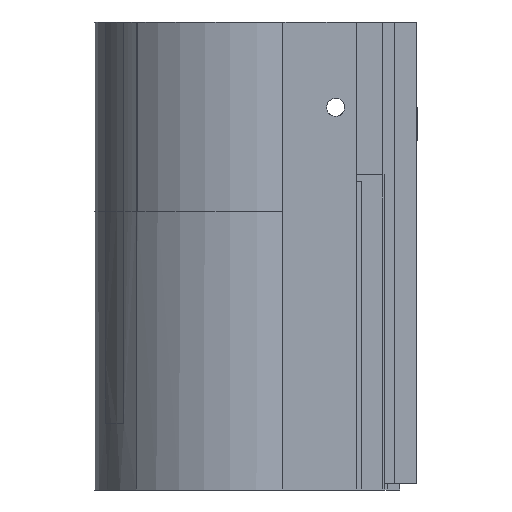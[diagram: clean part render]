
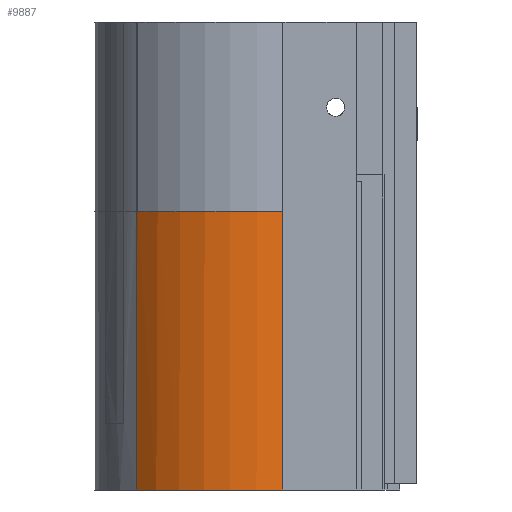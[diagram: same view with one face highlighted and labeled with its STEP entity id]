
A CAD part, left-side view. The second image highlights one B-rep face of the part: STEP entity #9887.
In plain terms, the highlighted cylindrical face has radius 25.3 mm (diameter 50.6 mm), a partial arc.
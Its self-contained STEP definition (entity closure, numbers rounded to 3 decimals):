
#1326 = CYLINDRICAL_SURFACE('',#1327,25.3);
#1327 = AXIS2_PLACEMENT_3D('',#1328,#1329,#1330);
#1328 = CARTESIAN_POINT('',(0.,17.3,45.));
#1329 = DIRECTION('',(0.,0.,1.));
#1330 = DIRECTION('',(1.,0.,0.));
#1355 = PLANE('',#1356);
#1356 = AXIS2_PLACEMENT_3D('',#1357,#1358,#1359);
#1357 = CARTESIAN_POINT('',(-11.232,-5.37,-1.));
#1358 = DIRECTION('',(0.,0.,1.));
#1359 = DIRECTION('',(1.,0.,0.));
#4476 = VERTEX_POINT('',#4477);
#4477 = CARTESIAN_POINT('',(-17.45,35.619,45.));
#4504 = EDGE_CURVE('',#4476,#4505,#4507,.T.);
#4505 = VERTEX_POINT('',#4506);
#4506 = CARTESIAN_POINT('',(-17.45,35.619,-1.));
#4507 = SURFACE_CURVE('',#4508,(#4512,#4519),.PCURVE_S1.);
#4508 = LINE('',#4509,#4510);
#4509 = CARTESIAN_POINT('',(-17.45,35.619,76.2));
#4510 = VECTOR('',#4511,1.);
#4511 = DIRECTION('',(0.,0.,-1.));
#4512 = PCURVE('',#1326,#4513);
#4513 = DEFINITIONAL_REPRESENTATION('',(#4514),#4518);
#4514 = LINE('',#4515,#4516);
#4515 = CARTESIAN_POINT('',(-3.951,31.2));
#4516 = VECTOR('',#4517,1.);
#4517 = DIRECTION('',(0.,-1.));
#4518 = ( GEOMETRIC_REPRESENTATION_CONTEXT(2) 
PARAMETRIC_REPRESENTATION_CONTEXT() REPRESENTATION_CONTEXT('2D SPACE',''
  ) );
#4519 = PCURVE('',#4520,#4525);
#4520 = CYLINDRICAL_SURFACE('',#4521,25.3);
#4521 = AXIS2_PLACEMENT_3D('',#4522,#4523,#4524);
#4522 = CARTESIAN_POINT('',(0.,17.3,45.));
#4523 = DIRECTION('',(0.,0.,1.));
#4524 = DIRECTION('',(1.,0.,0.));
#4525 = DEFINITIONAL_REPRESENTATION('',(#4526),#4530);
#4526 = LINE('',#4527,#4528);
#4527 = CARTESIAN_POINT('',(-3.951,31.2));
#4528 = VECTOR('',#4529,1.);
#4529 = DIRECTION('',(0.,-1.));
#4530 = ( GEOMETRIC_REPRESENTATION_CONTEXT(2) 
PARAMETRIC_REPRESENTATION_CONTEXT() REPRESENTATION_CONTEXT('2D SPACE',''
  ) );
#4862 = EDGE_CURVE('',#4863,#4505,#4865,.T.);
#4863 = VERTEX_POINT('',#4864);
#4864 = CARTESIAN_POINT('',(-24.618,11.467,-1.));
#4865 = SURFACE_CURVE('',#4866,(#4871,#4882),.PCURVE_S1.);
#4866 = CIRCLE('',#4867,25.3);
#4867 = AXIS2_PLACEMENT_3D('',#4868,#4869,#4870);
#4868 = CARTESIAN_POINT('',(0.,17.3,-1.));
#4869 = DIRECTION('',(0.,0.,-1.));
#4870 = DIRECTION('',(1.,0.,0.));
#4871 = PCURVE('',#1355,#4872);
#4872 = DEFINITIONAL_REPRESENTATION('',(#4873),#4881);
#4873 = ( BOUNDED_CURVE() B_SPLINE_CURVE(2,(#4874,#4875,#4876,#4877,
#4878,#4879,#4880),.UNSPECIFIED.,.T.,.F.) B_SPLINE_CURVE_WITH_KNOTS((1,2
    ,2,2,2,1),(-2.094,0.,2.094,4.189,
6.283,8.378),.UNSPECIFIED.) CURVE() 
GEOMETRIC_REPRESENTATION_ITEM() RATIONAL_B_SPLINE_CURVE((1.,0.5,1.,0.5,
1.,0.5,1.)) REPRESENTATION_ITEM('') );
#4874 = CARTESIAN_POINT('',(36.532,22.67));
#4875 = CARTESIAN_POINT('',(36.532,-21.151));
#4876 = CARTESIAN_POINT('',(-1.418,0.76));
#4877 = CARTESIAN_POINT('',(-39.368,22.67));
#4878 = CARTESIAN_POINT('',(-1.418,44.581));
#4879 = CARTESIAN_POINT('',(36.532,66.491));
#4880 = CARTESIAN_POINT('',(36.532,22.67));
#4881 = ( GEOMETRIC_REPRESENTATION_CONTEXT(2) 
PARAMETRIC_REPRESENTATION_CONTEXT() REPRESENTATION_CONTEXT('2D SPACE',''
  ) );
#4882 = PCURVE('',#4520,#4883);
#4883 = DEFINITIONAL_REPRESENTATION('',(#4884),#4888);
#4884 = LINE('',#4885,#4886);
#4885 = CARTESIAN_POINT('',(0.,-46.));
#4886 = VECTOR('',#4887,1.);
#4887 = DIRECTION('',(-1.,0.));
#4888 = ( GEOMETRIC_REPRESENTATION_CONTEXT(2) 
PARAMETRIC_REPRESENTATION_CONTEXT() REPRESENTATION_CONTEXT('2D SPACE',''
  ) );
#4906 = PLANE('',#4907);
#4907 = AXIS2_PLACEMENT_3D('',#4908,#4909,#4910);
#4908 = CARTESIAN_POINT('',(-11.993,11.467,-1.));
#4909 = DIRECTION('',(0.,-1.,0.));
#4910 = DIRECTION('',(-1.,0.,0.));
#9847 = CYLINDRICAL_SURFACE('',#9848,25.3);
#9848 = AXIS2_PLACEMENT_3D('',#9849,#9850,#9851);
#9849 = CARTESIAN_POINT('',(0.,17.3,45.));
#9850 = DIRECTION('',(0.,0.,-1.));
#9851 = DIRECTION('',(1.,0.,0.));
#9887 = ADVANCED_FACE('',(#9888),#4520,.T.);
#9888 = FACE_BOUND('',#9889,.F.);
#9889 = EDGE_LOOP('',(#9890,#9921,#9940,#9941,#9942));
#9890 = ORIENTED_EDGE('',*,*,#9891,.T.);
#9891 = EDGE_CURVE('',#9892,#9894,#9896,.T.);
#9892 = VERTEX_POINT('',#9893);
#9893 = CARTESIAN_POINT('',(-17.662,35.415,45.));
#9894 = VERTEX_POINT('',#9895);
#9895 = CARTESIAN_POINT('',(-24.618,11.467,45.));
#9896 = SURFACE_CURVE('',#9897,(#9902,#9909),.PCURVE_S1.);
#9897 = CIRCLE('',#9898,25.3);
#9898 = AXIS2_PLACEMENT_3D('',#9899,#9900,#9901);
#9899 = CARTESIAN_POINT('',(0.,17.3,45.));
#9900 = DIRECTION('',(0.,0.,1.));
#9901 = DIRECTION('',(1.,0.,0.));
#9902 = PCURVE('',#4520,#9903);
#9903 = DEFINITIONAL_REPRESENTATION('',(#9904),#9908);
#9904 = LINE('',#9905,#9906);
#9905 = CARTESIAN_POINT('',(-6.283,0.));
#9906 = VECTOR('',#9907,1.);
#9907 = DIRECTION('',(1.,0.));
#9908 = ( GEOMETRIC_REPRESENTATION_CONTEXT(2) 
PARAMETRIC_REPRESENTATION_CONTEXT() REPRESENTATION_CONTEXT('2D SPACE',''
  ) );
#9909 = PCURVE('',#9910,#9915);
#9910 = CYLINDRICAL_SURFACE('',#9911,25.3);
#9911 = AXIS2_PLACEMENT_3D('',#9912,#9913,#9914);
#9912 = CARTESIAN_POINT('',(0.,17.3,45.));
#9913 = DIRECTION('',(0.,0.,-1.));
#9914 = DIRECTION('',(1.,0.,0.));
#9915 = DEFINITIONAL_REPRESENTATION('',(#9916),#9920);
#9916 = LINE('',#9917,#9918);
#9917 = CARTESIAN_POINT('',(0.,0.));
#9918 = VECTOR('',#9919,1.);
#9919 = DIRECTION('',(-1.,0.));
#9920 = ( GEOMETRIC_REPRESENTATION_CONTEXT(2) 
PARAMETRIC_REPRESENTATION_CONTEXT() REPRESENTATION_CONTEXT('2D SPACE',''
  ) );
#9921 = ORIENTED_EDGE('',*,*,#9922,.F.);
#9922 = EDGE_CURVE('',#4863,#9894,#9923,.T.);
#9923 = SURFACE_CURVE('',#9924,(#9928,#9934),.PCURVE_S1.);
#9924 = LINE('',#9925,#9926);
#9925 = CARTESIAN_POINT('',(-24.618,11.467,45.));
#9926 = VECTOR('',#9927,1.);
#9927 = DIRECTION('',(0.,0.,1.));
#9928 = PCURVE('',#4520,#9929);
#9929 = DEFINITIONAL_REPRESENTATION('',(#9930),#9933);
#9930 = B_SPLINE_CURVE_WITH_KNOTS('',1,(#9931,#9932),.UNSPECIFIED.,.F.,
  .F.,(2,2),(-46.,0.),.PIECEWISE_BEZIER_KNOTS.);
#9931 = CARTESIAN_POINT('',(-2.909,-46.));
#9932 = CARTESIAN_POINT('',(-2.909,0.));
#9933 = ( GEOMETRIC_REPRESENTATION_CONTEXT(2) 
PARAMETRIC_REPRESENTATION_CONTEXT() REPRESENTATION_CONTEXT('2D SPACE',''
  ) );
#9934 = PCURVE('',#4906,#9935);
#9935 = DEFINITIONAL_REPRESENTATION('',(#9936),#9939);
#9936 = B_SPLINE_CURVE_WITH_KNOTS('',1,(#9937,#9938),.UNSPECIFIED.,.F.,
  .F.,(2,2),(-46.,0.),.PIECEWISE_BEZIER_KNOTS.);
#9937 = CARTESIAN_POINT('',(12.625,0.));
#9938 = CARTESIAN_POINT('',(12.625,-46.));
#9939 = ( GEOMETRIC_REPRESENTATION_CONTEXT(2) 
PARAMETRIC_REPRESENTATION_CONTEXT() REPRESENTATION_CONTEXT('2D SPACE',''
  ) );
#9940 = ORIENTED_EDGE('',*,*,#4862,.T.);
#9941 = ORIENTED_EDGE('',*,*,#4504,.F.);
#9942 = ORIENTED_EDGE('',*,*,#9943,.T.);
#9943 = EDGE_CURVE('',#4476,#9892,#9944,.T.);
#9944 = SURFACE_CURVE('',#9945,(#9950,#9957),.PCURVE_S1.);
#9945 = CIRCLE('',#9946,25.3);
#9946 = AXIS2_PLACEMENT_3D('',#9947,#9948,#9949);
#9947 = CARTESIAN_POINT('',(0.,17.3,45.));
#9948 = DIRECTION('',(0.,0.,1.));
#9949 = DIRECTION('',(1.,0.,0.));
#9950 = PCURVE('',#4520,#9951);
#9951 = DEFINITIONAL_REPRESENTATION('',(#9952),#9956);
#9952 = LINE('',#9953,#9954);
#9953 = CARTESIAN_POINT('',(-6.283,0.));
#9954 = VECTOR('',#9955,1.);
#9955 = DIRECTION('',(1.,0.));
#9956 = ( GEOMETRIC_REPRESENTATION_CONTEXT(2) 
PARAMETRIC_REPRESENTATION_CONTEXT() REPRESENTATION_CONTEXT('2D SPACE',''
  ) );
#9957 = PCURVE('',#9847,#9958);
#9958 = DEFINITIONAL_REPRESENTATION('',(#9959),#9963);
#9959 = LINE('',#9960,#9961);
#9960 = CARTESIAN_POINT('',(0.,0.));
#9961 = VECTOR('',#9962,1.);
#9962 = DIRECTION('',(-1.,0.));
#9963 = ( GEOMETRIC_REPRESENTATION_CONTEXT(2) 
PARAMETRIC_REPRESENTATION_CONTEXT() REPRESENTATION_CONTEXT('2D SPACE',''
  ) );
